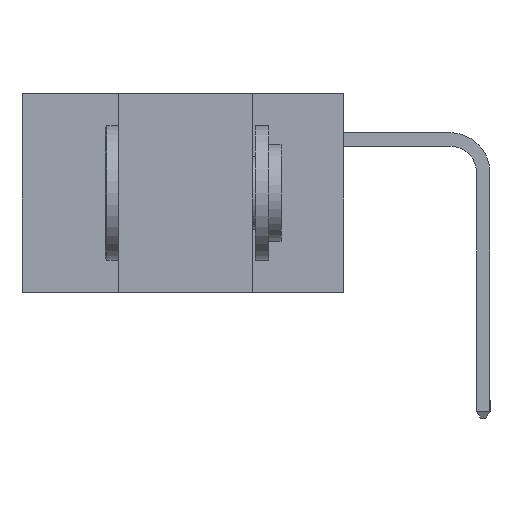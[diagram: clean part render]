
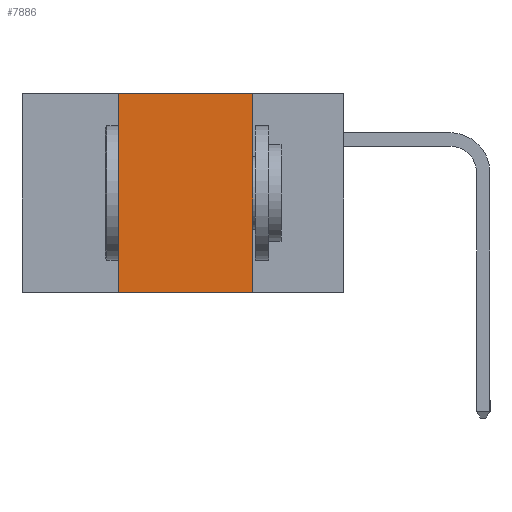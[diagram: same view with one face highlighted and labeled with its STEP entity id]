
A CAD part, left-side view. The second image highlights one B-rep face of the part: STEP entity #7886.
In plain terms, the highlighted planar face has unit normal (-1, 0, 0).
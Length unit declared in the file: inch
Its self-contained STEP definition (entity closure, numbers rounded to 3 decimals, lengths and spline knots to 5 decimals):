
#706 = CARTESIAN_POINT ( 'NONE',  ( 0., 0.42, 0. ) ) ;
#894 = DIRECTION ( 'NONE',  ( 0., -1., 0. ) ) ;
#1124 = ORIENTED_EDGE ( 'NONE', *, *, #9526, .T. ) ;
#1670 = CARTESIAN_POINT ( 'NONE',  ( 0., 0.6, 0. ) ) ;
#2277 = VERTEX_POINT ( 'NONE', #3818 ) ;
#2321 = VECTOR ( 'NONE', #10543, 39.37008 ) ;
#3603 = CARTESIAN_POINT ( 'NONE',  ( 0., 0.17, -0.37 ) ) ;
#3818 = CARTESIAN_POINT ( 'NONE',  ( 0., 0.17, -0.37 ) ) ;
#4712 = PLANE ( 'NONE',  #10931 ) ;
#4750 = DIRECTION ( 'NONE',  ( 0., 0., -1. ) ) ;
#4805 = VERTEX_POINT ( 'NONE', #13025 ) ;
#4895 = VECTOR ( 'NONE', #894, 39.37008 ) ;
#5203 = LINE ( 'NONE', #11975, #4895 ) ;
#5465 = DIRECTION ( 'NONE',  ( 0., 0., 1. ) ) ;
#5925 = VERTEX_POINT ( 'NONE', #6763 ) ;
#6250 = ORIENTED_EDGE ( 'NONE', *, *, #11525, .F. ) ;
#6763 = CARTESIAN_POINT ( 'NONE',  ( 0., 0.17, 0. ) ) ;
#6779 = VECTOR ( 'NONE', #9318, 39.37008 ) ;
#7886 = ADVANCED_FACE ( 'NONE', ( #10195 ), #4712, .F. ) ;
#8904 = ORIENTED_EDGE ( 'NONE', *, *, #10850, .F. ) ;
#8947 = VECTOR ( 'NONE', #5465, 39.37008 ) ;
#9318 = DIRECTION ( 'NONE',  ( 0., -1., 0. ) ) ;
#9383 = LINE ( 'NONE', #11277, #6779 ) ;
#9526 = EDGE_CURVE ( 'NONE', #4805, #2277, #5203, .T. ) ;
#9596 = EDGE_LOOP ( 'NONE', ( #6250, #8904, #11533, #1124 ) ) ;
#10179 = EDGE_CURVE ( 'NONE', #4805, #10538, #11570, .T. ) ;
#10195 = FACE_OUTER_BOUND ( 'NONE', #9596, .T. ) ;
#10538 = VERTEX_POINT ( 'NONE', #706 ) ;
#10543 = DIRECTION ( 'NONE',  ( 0., 0., -1. ) ) ;
#10703 = DIRECTION ( 'NONE',  ( 1., 0., 0. ) ) ;
#10850 = EDGE_CURVE ( 'NONE', #10538, #5925, #9383, .T. ) ;
#10931 = AXIS2_PLACEMENT_3D ( 'NONE', #1670, #10703, #4750 ) ;
#11277 = CARTESIAN_POINT ( 'NONE',  ( 0., 0.6, 0. ) ) ;
#11525 = EDGE_CURVE ( 'NONE', #5925, #2277, #12884, .T. ) ;
#11533 = ORIENTED_EDGE ( 'NONE', *, *, #10179, .F. ) ;
#11570 = LINE ( 'NONE', #12400, #8947 ) ;
#11975 = CARTESIAN_POINT ( 'NONE',  ( 0., 0.6, -0.37 ) ) ;
#12400 = CARTESIAN_POINT ( 'NONE',  ( 0., 0.42, -0.37 ) ) ;
#12884 = LINE ( 'NONE', #3603, #2321 ) ;
#13025 = CARTESIAN_POINT ( 'NONE',  ( 0., 0.42, -0.37 ) ) ;
